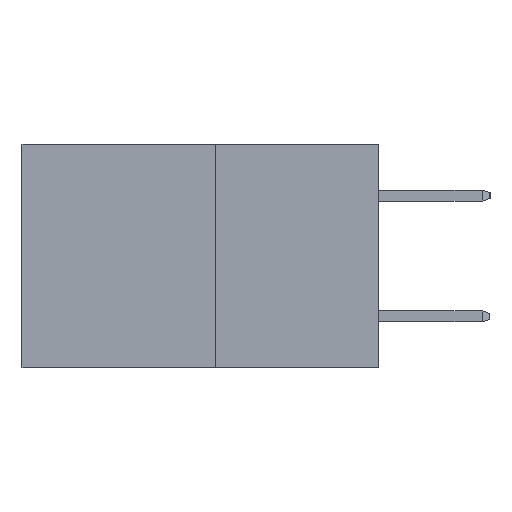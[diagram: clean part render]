
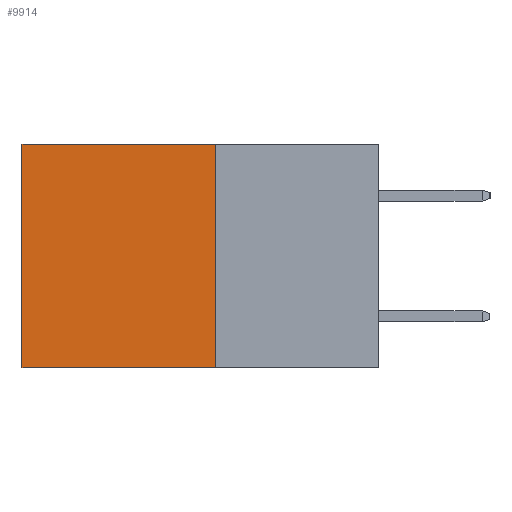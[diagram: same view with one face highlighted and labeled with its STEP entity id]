
A CAD part, left-side view. The second image highlights one B-rep face of the part: STEP entity #9914.
In plain terms, the highlighted planar face has unit normal (-1, 0, 0).
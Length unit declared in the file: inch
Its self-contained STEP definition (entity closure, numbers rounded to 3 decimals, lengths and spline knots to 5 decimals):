
#104 = VECTOR ( 'NONE', #952, 39.37008 ) ;
#684 = CARTESIAN_POINT ( 'NONE',  ( 0.277, 0.27, 0. ) ) ;
#803 = CARTESIAN_POINT ( 'NONE',  ( 0.277, 0.59, -0.37 ) ) ;
#952 = DIRECTION ( 'NONE',  ( 0., 1., 0. ) ) ;
#1754 = CARTESIAN_POINT ( 'NONE',  ( 0.277, 0.27, -0.37 ) ) ;
#1948 = DIRECTION ( 'NONE',  ( 0., 0., -1. ) ) ;
#1967 = DIRECTION ( 'NONE',  ( 1., 0., 0. ) ) ;
#2040 = EDGE_CURVE ( 'NONE', #16698, #5570, #16999, .T. ) ;
#2578 = EDGE_CURVE ( 'NONE', #19566, #6898, #7006, .T. ) ;
#4351 = ORIENTED_EDGE ( 'NONE', *, *, #2578, .T. ) ;
#4398 = CARTESIAN_POINT ( 'NONE',  ( 0.277, 0.27, -0.37 ) ) ;
#5329 = LINE ( 'NONE', #4398, #104 ) ;
#5570 = VERTEX_POINT ( 'NONE', #17728 ) ;
#6898 = VERTEX_POINT ( 'NONE', #9667 ) ;
#7006 = LINE ( 'NONE', #803, #7543 ) ;
#7543 = VECTOR ( 'NONE', #19353, 39.37008 ) ;
#8513 = ORIENTED_EDGE ( 'NONE', *, *, #2040, .F. ) ;
#9667 = CARTESIAN_POINT ( 'NONE',  ( 0.277, 0.59, -0.37 ) ) ;
#9684 = LINE ( 'NONE', #14772, #18388 ) ;
#9765 = AXIS2_PLACEMENT_3D ( 'NONE', #12380, #1967, #14134 ) ;
#9914 = ADVANCED_FACE ( 'NONE', ( #17226 ), #21032, .F. ) ;
#10523 = EDGE_CURVE ( 'NONE', #5570, #6898, #5329, .T. ) ;
#12380 = CARTESIAN_POINT ( 'NONE',  ( 0.277, 0.27, -0.37 ) ) ;
#12404 = VECTOR ( 'NONE', #1948, 39.37008 ) ;
#14134 = DIRECTION ( 'NONE',  ( 0., 0., -1. ) ) ;
#14772 = CARTESIAN_POINT ( 'NONE',  ( 0.277, 0.27, 0. ) ) ;
#15606 = EDGE_CURVE ( 'NONE', #16698, #19566, #9684, .T. ) ;
#16507 = DIRECTION ( 'NONE',  ( 0., 1., 0. ) ) ;
#16698 = VERTEX_POINT ( 'NONE', #684 ) ;
#16999 = LINE ( 'NONE', #1754, #12404 ) ;
#17226 = FACE_OUTER_BOUND ( 'NONE', #19932, .T. ) ;
#17536 = ORIENTED_EDGE ( 'NONE', *, *, #10523, .F. ) ;
#17728 = CARTESIAN_POINT ( 'NONE',  ( 0.277, 0.27, -0.37 ) ) ;
#18388 = VECTOR ( 'NONE', #16507, 39.37008 ) ;
#18890 = CARTESIAN_POINT ( 'NONE',  ( 0.277, 0.59, 0. ) ) ;
#19353 = DIRECTION ( 'NONE',  ( 0., 0., -1. ) ) ;
#19566 = VERTEX_POINT ( 'NONE', #18890 ) ;
#19932 = EDGE_LOOP ( 'NONE', ( #4351, #17536, #8513, #22379 ) ) ;
#21032 = PLANE ( 'NONE',  #9765 ) ;
#22379 = ORIENTED_EDGE ( 'NONE', *, *, #15606, .T. ) ;
